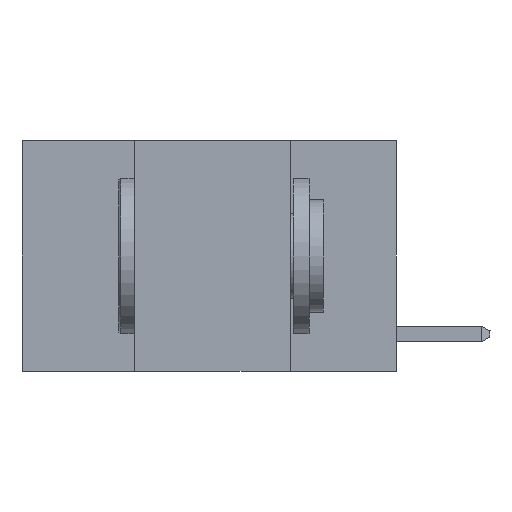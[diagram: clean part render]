
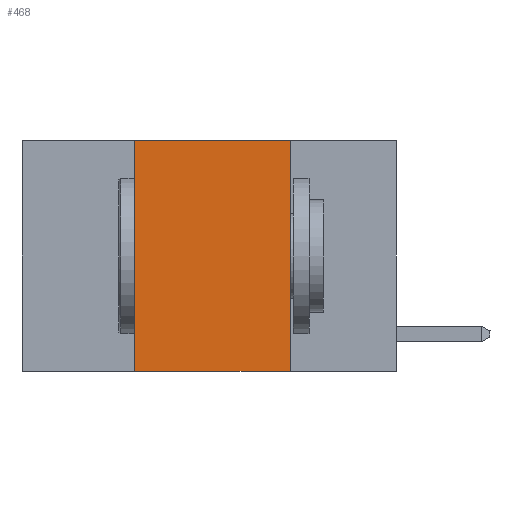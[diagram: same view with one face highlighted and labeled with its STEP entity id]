
A CAD part, left-side view. The second image highlights one B-rep face of the part: STEP entity #468.
In plain terms, the highlighted planar face has unit normal (-1, 0, 0).
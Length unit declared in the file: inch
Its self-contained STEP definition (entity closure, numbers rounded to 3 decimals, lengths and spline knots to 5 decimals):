
#46 = VECTOR ( 'NONE', #1031, 39.37008 ) ;
#468 = ADVANCED_FACE ( 'NONE', ( #5571 ), #18235, .F. ) ;
#943 = VERTEX_POINT ( 'NONE', #13807 ) ;
#1018 = DIRECTION ( 'NONE',  ( 0., 0., -1. ) ) ;
#1031 = DIRECTION ( 'NONE',  ( 0., -1., 0. ) ) ;
#1207 = CARTESIAN_POINT ( 'NONE',  ( 0., 0.17, 0. ) ) ;
#1287 = LINE ( 'NONE', #6035, #18713 ) ;
#1781 = EDGE_CURVE ( 'NONE', #6541, #943, #14689, .T. ) ;
#1995 = VECTOR ( 'NONE', #11970, 39.37008 ) ;
#2733 = LINE ( 'NONE', #1207, #1995 ) ;
#3156 = VECTOR ( 'NONE', #16254, 39.37008 ) ;
#3697 = EDGE_CURVE ( 'NONE', #943, #13716, #2733, .T. ) ;
#3826 = VERTEX_POINT ( 'NONE', #12365 ) ;
#4056 = ORIENTED_EDGE ( 'NONE', *, *, #7339, .F. ) ;
#5571 = FACE_OUTER_BOUND ( 'NONE', #5904, .T. ) ;
#5904 = EDGE_LOOP ( 'NONE', ( #17868, #14230, #4056, #13434 ) ) ;
#6035 = CARTESIAN_POINT ( 'NONE',  ( 0., 0.42, 0. ) ) ;
#6541 = VERTEX_POINT ( 'NONE', #14287 ) ;
#7339 = EDGE_CURVE ( 'NONE', #3826, #6541, #1287, .T. ) ;
#7787 = DIRECTION ( 'NONE',  ( 0., 0., 1. ) ) ;
#10231 = CARTESIAN_POINT ( 'NONE',  ( 0., 0.6, 0. ) ) ;
#10540 = DIRECTION ( 'NONE',  ( 1., 0., 0. ) ) ;
#11421 = AXIS2_PLACEMENT_3D ( 'NONE', #10231, #10540, #1018 ) ;
#11970 = DIRECTION ( 'NONE',  ( 0., 0., -1. ) ) ;
#12206 = CARTESIAN_POINT ( 'NONE',  ( 0., 0.6, -0.37 ) ) ;
#12365 = CARTESIAN_POINT ( 'NONE',  ( 0., 0.42, -0.37 ) ) ;
#13434 = ORIENTED_EDGE ( 'NONE', *, *, #20353, .T. ) ;
#13716 = VERTEX_POINT ( 'NONE', #18891 ) ;
#13807 = CARTESIAN_POINT ( 'NONE',  ( 0., 0.17, 0. ) ) ;
#14230 = ORIENTED_EDGE ( 'NONE', *, *, #1781, .F. ) ;
#14287 = CARTESIAN_POINT ( 'NONE',  ( 0., 0.42, 0. ) ) ;
#14689 = LINE ( 'NONE', #18139, #3156 ) ;
#16254 = DIRECTION ( 'NONE',  ( 0., -1., 0. ) ) ;
#16585 = LINE ( 'NONE', #12206, #46 ) ;
#17868 = ORIENTED_EDGE ( 'NONE', *, *, #3697, .F. ) ;
#18139 = CARTESIAN_POINT ( 'NONE',  ( 0., 0.6, 0. ) ) ;
#18235 = PLANE ( 'NONE',  #11421 ) ;
#18713 = VECTOR ( 'NONE', #7787, 39.37008 ) ;
#18891 = CARTESIAN_POINT ( 'NONE',  ( 0., 0.17, -0.37 ) ) ;
#20353 = EDGE_CURVE ( 'NONE', #3826, #13716, #16585, .T. ) ;
